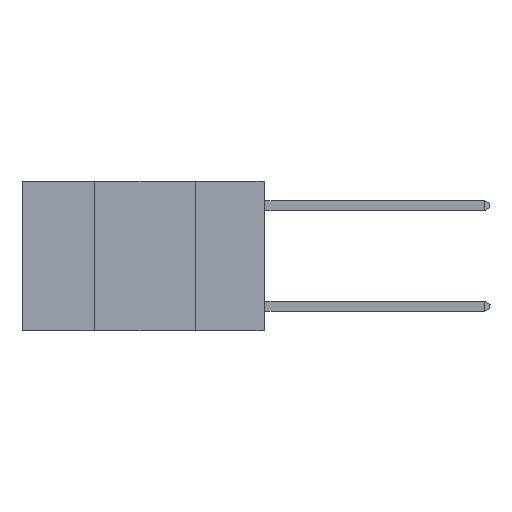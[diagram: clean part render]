
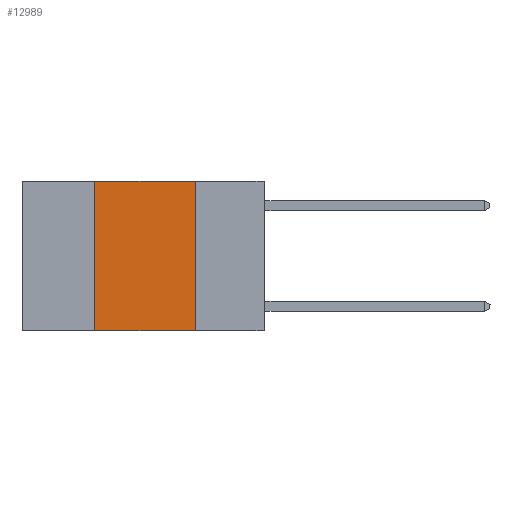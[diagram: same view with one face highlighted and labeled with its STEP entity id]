
A CAD part, left-side view. The second image highlights one B-rep face of the part: STEP entity #12989.
In plain terms, the highlighted planar face has unit normal (-1, 0, 0).
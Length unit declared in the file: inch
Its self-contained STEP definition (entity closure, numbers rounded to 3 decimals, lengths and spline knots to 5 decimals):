
#253 = EDGE_CURVE ( 'NONE', #12594, #3238, #10398, .T. ) ;
#820 = EDGE_CURVE ( 'NONE', #3238, #11769, #21728, .T. ) ;
#1380 = PLANE ( 'NONE',  #2824 ) ;
#1623 = FACE_OUTER_BOUND ( 'NONE', #10444, .T. ) ;
#1715 = LINE ( 'NONE', #15882, #26681 ) ;
#1759 = DIRECTION ( 'NONE',  ( 0., 0., 1. ) ) ;
#2117 = ORIENTED_EDGE ( 'NONE', *, *, #253, .F. ) ;
#2233 = CARTESIAN_POINT ( 'NONE',  ( 0., 0.17, 0. ) ) ;
#2824 = AXIS2_PLACEMENT_3D ( 'NONE', #25559, #3853, #20905 ) ;
#3071 = EDGE_CURVE ( 'NONE', #11441, #12594, #30455, .T. ) ;
#3238 = VERTEX_POINT ( 'NONE', #26490 ) ;
#3853 = DIRECTION ( 'NONE',  ( 1., 0., 0. ) ) ;
#4451 = CARTESIAN_POINT ( 'NONE',  ( 0., 0.17, -0.37 ) ) ;
#6207 = DIRECTION ( 'NONE',  ( 0., -1., 0. ) ) ;
#10398 = LINE ( 'NONE', #12328, #29477 ) ;
#10444 = EDGE_LOOP ( 'NONE', ( #17287, #2117, #12848, #27020 ) ) ;
#10869 = EDGE_CURVE ( 'NONE', #11441, #11769, #1715, .T. ) ;
#11441 = VERTEX_POINT ( 'NONE', #20262 ) ;
#11769 = VERTEX_POINT ( 'NONE', #4451 ) ;
#12328 = CARTESIAN_POINT ( 'NONE',  ( 0., 0.6, 0. ) ) ;
#12594 = VERTEX_POINT ( 'NONE', #14567 ) ;
#12848 = ORIENTED_EDGE ( 'NONE', *, *, #3071, .F. ) ;
#12989 = ADVANCED_FACE ( 'NONE', ( #1623 ), #1380, .F. ) ;
#14567 = CARTESIAN_POINT ( 'NONE',  ( 0., 0.42, 0. ) ) ;
#15882 = CARTESIAN_POINT ( 'NONE',  ( 0., 0.6, -0.37 ) ) ;
#16386 = CARTESIAN_POINT ( 'NONE',  ( 0., 0.42, 0. ) ) ;
#16804 = VECTOR ( 'NONE', #19296, 39.37008 ) ;
#17287 = ORIENTED_EDGE ( 'NONE', *, *, #820, .F. ) ;
#19296 = DIRECTION ( 'NONE',  ( 0., 0., -1. ) ) ;
#19383 = VECTOR ( 'NONE', #1759, 39.37008 ) ;
#20262 = CARTESIAN_POINT ( 'NONE',  ( 0., 0.42, -0.37 ) ) ;
#20905 = DIRECTION ( 'NONE',  ( 0., 0., -1. ) ) ;
#21728 = LINE ( 'NONE', #2233, #16804 ) ;
#25559 = CARTESIAN_POINT ( 'NONE',  ( 0., 0.6, 0. ) ) ;
#26490 = CARTESIAN_POINT ( 'NONE',  ( 0., 0.17, 0. ) ) ;
#26681 = VECTOR ( 'NONE', #6207, 39.37008 ) ;
#27020 = ORIENTED_EDGE ( 'NONE', *, *, #10869, .T. ) ;
#29028 = DIRECTION ( 'NONE',  ( 0., -1., 0. ) ) ;
#29477 = VECTOR ( 'NONE', #29028, 39.37008 ) ;
#30455 = LINE ( 'NONE', #16386, #19383 ) ;
